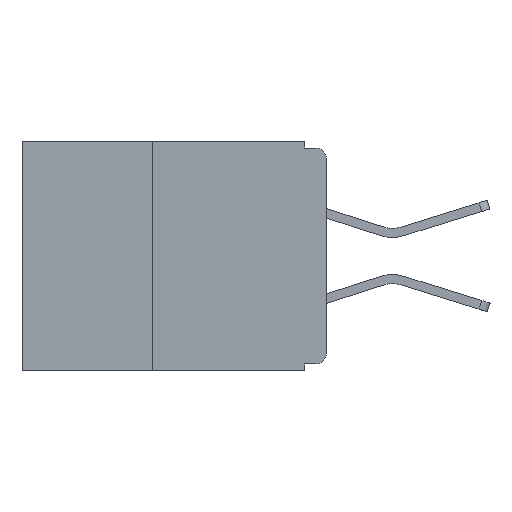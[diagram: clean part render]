
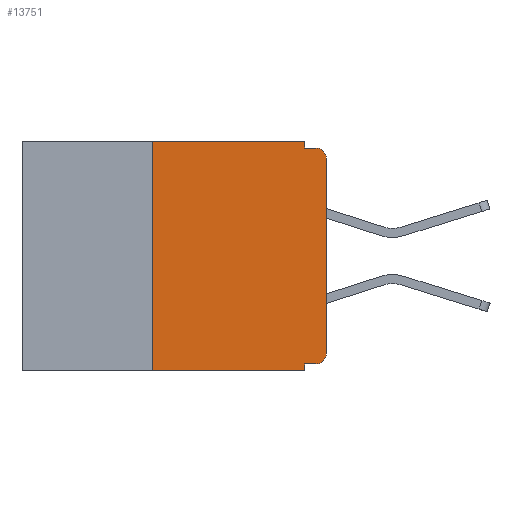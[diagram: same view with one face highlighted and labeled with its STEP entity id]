
A CAD part, left-side view. The second image highlights one B-rep face of the part: STEP entity #13751.
In plain terms, the highlighted planar face has unit normal (-1, 0, 0).
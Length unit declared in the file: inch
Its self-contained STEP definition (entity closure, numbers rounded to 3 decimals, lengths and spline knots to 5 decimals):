
#41 = CARTESIAN_POINT ( 'NONE',  ( 0., 0.031, 0. ) ) ;
#285 = EDGE_CURVE ( 'NONE', #5811, #5631, #3807, .T. ) ;
#614 = CARTESIAN_POINT ( 'NONE',  ( 0., 0., -0.305 ) ) ;
#620 = CIRCLE ( 'NONE', #2297, 0.015 ) ;
#930 = ORIENTED_EDGE ( 'NONE', *, *, #3962, .T. ) ;
#1196 = EDGE_CURVE ( 'NONE', #14784, #13942, #16410, .T. ) ;
#1225 = CARTESIAN_POINT ( 'NONE',  ( 0., 0.437, -0.33 ) ) ;
#1254 = LINE ( 'NONE', #1225, #14038 ) ;
#1652 = DIRECTION ( 'NONE',  ( 1., 0., 0. ) ) ;
#2175 = DIRECTION ( 'NONE',  ( -1., 0., 0. ) ) ;
#2190 = AXIS2_PLACEMENT_3D ( 'NONE', #9394, #1652, #10682 ) ;
#2202 = CARTESIAN_POINT ( 'NONE',  ( 0., 0.015, -0.32 ) ) ;
#2297 = AXIS2_PLACEMENT_3D ( 'NONE', #6842, #5946, #8369 ) ;
#2808 = ORIENTED_EDGE ( 'NONE', *, *, #16409, .T. ) ;
#2817 = CARTESIAN_POINT ( 'NONE',  ( 0., 0.25, 0. ) ) ;
#3068 = ORIENTED_EDGE ( 'NONE', *, *, #285, .F. ) ;
#3138 = CARTESIAN_POINT ( 'NONE',  ( 0., 0.25, -0.33 ) ) ;
#3379 = CARTESIAN_POINT ( 'NONE',  ( 0., 0.031, -0.33 ) ) ;
#3385 = EDGE_CURVE ( 'NONE', #14436, #7464, #620, .T. ) ;
#3468 = CARTESIAN_POINT ( 'NONE',  ( 0., 0.031, -0.32 ) ) ;
#3483 = ORIENTED_EDGE ( 'NONE', *, *, #7730, .F. ) ;
#3595 = DIRECTION ( 'NONE',  ( 0., -1., 0. ) ) ;
#3807 = LINE ( 'NONE', #9273, #16444 ) ;
#3932 = CARTESIAN_POINT ( 'NONE',  ( 0., 0.015, -0.01 ) ) ;
#3962 = EDGE_CURVE ( 'NONE', #5890, #14436, #5940, .T. ) ;
#4221 = CARTESIAN_POINT ( 'NONE',  ( 0., 0.031, -0.33 ) ) ;
#4233 = AXIS2_PLACEMENT_3D ( 'NONE', #9912, #2175, #11193 ) ;
#4551 = ORIENTED_EDGE ( 'NONE', *, *, #14352, .F. ) ;
#4712 = LINE ( 'NONE', #5244, #11488 ) ;
#5149 = CIRCLE ( 'NONE', #4233, 0.015 ) ;
#5244 = CARTESIAN_POINT ( 'NONE',  ( 0., 0.437, 0. ) ) ;
#5631 = VERTEX_POINT ( 'NONE', #2817 ) ;
#5641 = CARTESIAN_POINT ( 'NONE',  ( 0., 0., -0.025 ) ) ;
#5811 = VERTEX_POINT ( 'NONE', #3138 ) ;
#5890 = VERTEX_POINT ( 'NONE', #614 ) ;
#5940 = LINE ( 'NONE', #12135, #15583 ) ;
#5946 = DIRECTION ( 'NONE',  ( -1., 0., 0. ) ) ;
#6842 = CARTESIAN_POINT ( 'NONE',  ( 0., 0.015, -0.025 ) ) ;
#7042 = ORIENTED_EDGE ( 'NONE', *, *, #3385, .T. ) ;
#7400 = FACE_OUTER_BOUND ( 'NONE', #9591, .T. ) ;
#7464 = VERTEX_POINT ( 'NONE', #3932 ) ;
#7730 = EDGE_CURVE ( 'NONE', #15395, #11749, #13480, .T. ) ;
#8316 = DIRECTION ( 'NONE',  ( 0., 0., 1. ) ) ;
#8327 = ORIENTED_EDGE ( 'NONE', *, *, #16000, .T. ) ;
#8369 = DIRECTION ( 'NONE',  ( 0., 0., -1. ) ) ;
#8483 = CARTESIAN_POINT ( 'NONE',  ( 0., 0.031, -0.01 ) ) ;
#9273 = CARTESIAN_POINT ( 'NONE',  ( 0., 0.25, -0.33 ) ) ;
#9394 = CARTESIAN_POINT ( 'NONE',  ( 0., 0.437, 0. ) ) ;
#9591 = EDGE_LOOP ( 'NONE', ( #930, #7042, #10626, #11314, #14708, #3068, #8327, #4551, #3483, #2808 ) ) ;
#9912 = CARTESIAN_POINT ( 'NONE',  ( 0., 0.015, -0.305 ) ) ;
#9925 = DIRECTION ( 'NONE',  ( 0., 0., 1. ) ) ;
#10236 = VECTOR ( 'NONE', #3595, 39.37008 ) ;
#10257 = DIRECTION ( 'NONE',  ( 0., -1., 0. ) ) ;
#10622 = PLANE ( 'NONE',  #2190 ) ;
#10626 = ORIENTED_EDGE ( 'NONE', *, *, #12809, .F. ) ;
#10682 = DIRECTION ( 'NONE',  ( 0., 0., -1. ) ) ;
#10826 = EDGE_CURVE ( 'NONE', #5631, #14784, #4712, .T. ) ;
#11193 = DIRECTION ( 'NONE',  ( 0., 0., -1. ) ) ;
#11314 = ORIENTED_EDGE ( 'NONE', *, *, #1196, .F. ) ;
#11315 = CARTESIAN_POINT ( 'NONE',  ( 0., 0., -0.01 ) ) ;
#11467 = DIRECTION ( 'NONE',  ( 0., 1., 0. ) ) ;
#11488 = VECTOR ( 'NONE', #16483, 39.37008 ) ;
#11490 = DIRECTION ( 'NONE',  ( 0., 0., -1. ) ) ;
#11749 = VERTEX_POINT ( 'NONE', #3468 ) ;
#11989 = VECTOR ( 'NONE', #13093, 39.37008 ) ;
#12135 = CARTESIAN_POINT ( 'NONE',  ( 0., 0., 0. ) ) ;
#12749 = VERTEX_POINT ( 'NONE', #3379 ) ;
#12779 = LINE ( 'NONE', #11315, #10236 ) ;
#12781 = CARTESIAN_POINT ( 'NONE',  ( 0., 0., -0.32 ) ) ;
#12809 = EDGE_CURVE ( 'NONE', #13942, #7464, #12779, .T. ) ;
#13093 = DIRECTION ( 'NONE',  ( 0., 0., -1. ) ) ;
#13106 = VECTOR ( 'NONE', #11467, 39.37008 ) ;
#13142 = VECTOR ( 'NONE', #11490, 39.37008 ) ;
#13480 = LINE ( 'NONE', #12781, #13106 ) ;
#13751 = ADVANCED_FACE ( 'NONE', ( #7400 ), #10622, .F. ) ;
#13942 = VERTEX_POINT ( 'NONE', #8483 ) ;
#14038 = VECTOR ( 'NONE', #10257, 39.37008 ) ;
#14352 = EDGE_CURVE ( 'NONE', #11749, #12749, #15281, .T. ) ;
#14436 = VERTEX_POINT ( 'NONE', #5641 ) ;
#14708 = ORIENTED_EDGE ( 'NONE', *, *, #10826, .F. ) ;
#14784 = VERTEX_POINT ( 'NONE', #41 ) ;
#15281 = LINE ( 'NONE', #4221, #11989 ) ;
#15304 = CARTESIAN_POINT ( 'NONE',  ( 0., 0.031, 0. ) ) ;
#15395 = VERTEX_POINT ( 'NONE', #2202 ) ;
#15583 = VECTOR ( 'NONE', #9925, 39.37008 ) ;
#16000 = EDGE_CURVE ( 'NONE', #5811, #12749, #1254, .T. ) ;
#16409 = EDGE_CURVE ( 'NONE', #15395, #5890, #5149, .T. ) ;
#16410 = LINE ( 'NONE', #15304, #13142 ) ;
#16444 = VECTOR ( 'NONE', #8316, 39.37008 ) ;
#16483 = DIRECTION ( 'NONE',  ( 0., -1., 0. ) ) ;
